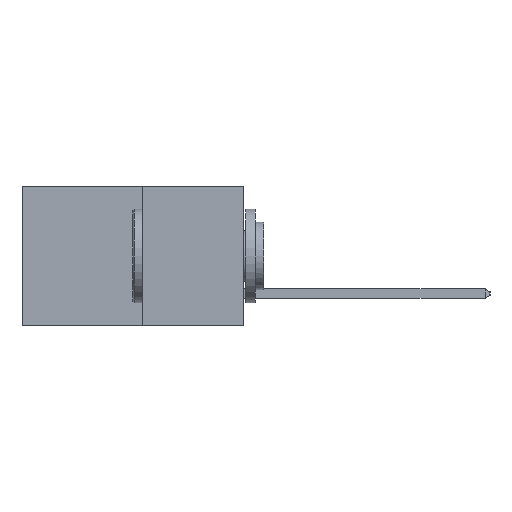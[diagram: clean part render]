
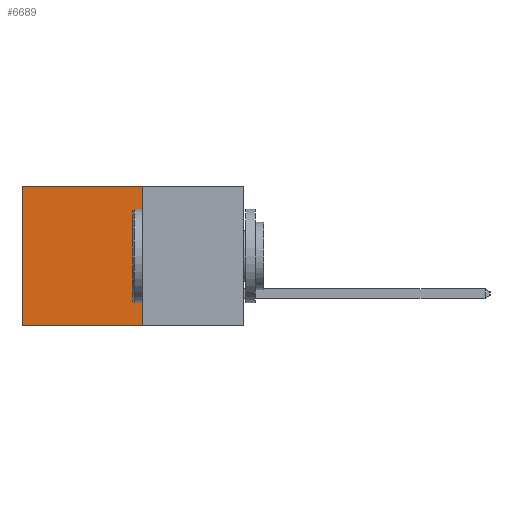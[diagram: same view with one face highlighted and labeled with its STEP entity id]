
A CAD part, left-side view. The second image highlights one B-rep face of the part: STEP entity #6689.
In plain terms, the highlighted planar face has unit normal (-1, 0, 0).
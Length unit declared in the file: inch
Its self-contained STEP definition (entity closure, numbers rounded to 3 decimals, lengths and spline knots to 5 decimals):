
#258 = ORIENTED_EDGE ( 'NONE', *, *, #5710, .T. ) ;
#712 = VERTEX_POINT ( 'NONE', #10095 ) ;
#1313 = VECTOR ( 'NONE', #12692, 39.37008 ) ;
#1452 = CARTESIAN_POINT ( 'NONE',  ( 0.277, 0.27, -0.37 ) ) ;
#1716 = ORIENTED_EDGE ( 'NONE', *, *, #10541, .F. ) ;
#2598 = ORIENTED_EDGE ( 'NONE', *, *, #6685, .F. ) ;
#3275 = VERTEX_POINT ( 'NONE', #8425 ) ;
#3766 = VERTEX_POINT ( 'NONE', #10313 ) ;
#3911 = DIRECTION ( 'NONE',  ( 1., 0., 0. ) ) ;
#4015 = PLANE ( 'NONE',  #11000 ) ;
#4026 = CARTESIAN_POINT ( 'NONE',  ( 0.277, 0.27, -0.37 ) ) ;
#4222 = DIRECTION ( 'NONE',  ( 0., 0., -1. ) ) ;
#4405 = CARTESIAN_POINT ( 'NONE',  ( 0.277, 0.27, -0.37 ) ) ;
#5164 = LINE ( 'NONE', #4405, #10307 ) ;
#5267 = VERTEX_POINT ( 'NONE', #11724 ) ;
#5359 = LINE ( 'NONE', #9083, #7827 ) ;
#5710 = EDGE_CURVE ( 'NONE', #712, #3275, #5359, .T. ) ;
#6685 = EDGE_CURVE ( 'NONE', #5267, #3766, #5164, .T. ) ;
#6689 = ADVANCED_FACE ( 'NONE', ( #12593 ), #4015, .F. ) ;
#6745 = DIRECTION ( 'NONE',  ( 0., 0., -1. ) ) ;
#6902 = LINE ( 'NONE', #12719, #9647 ) ;
#7827 = VECTOR ( 'NONE', #9315, 39.37008 ) ;
#7901 = EDGE_LOOP ( 'NONE', ( #258, #1716, #2598, #11240 ) ) ;
#8425 = CARTESIAN_POINT ( 'NONE',  ( 0.277, 0.59, -0.37 ) ) ;
#9083 = CARTESIAN_POINT ( 'NONE',  ( 0.277, 0.59, -0.37 ) ) ;
#9272 = EDGE_CURVE ( 'NONE', #5267, #712, #6902, .T. ) ;
#9315 = DIRECTION ( 'NONE',  ( 0., 0., -1. ) ) ;
#9610 = LINE ( 'NONE', #1452, #1313 ) ;
#9647 = VECTOR ( 'NONE', #10763, 39.37008 ) ;
#10095 = CARTESIAN_POINT ( 'NONE',  ( 0.277, 0.59, 0. ) ) ;
#10307 = VECTOR ( 'NONE', #4222, 39.37008 ) ;
#10313 = CARTESIAN_POINT ( 'NONE',  ( 0.277, 0.27, -0.37 ) ) ;
#10541 = EDGE_CURVE ( 'NONE', #3766, #3275, #9610, .T. ) ;
#10763 = DIRECTION ( 'NONE',  ( 0., 1., 0. ) ) ;
#11000 = AXIS2_PLACEMENT_3D ( 'NONE', #4026, #3911, #6745 ) ;
#11240 = ORIENTED_EDGE ( 'NONE', *, *, #9272, .T. ) ;
#11724 = CARTESIAN_POINT ( 'NONE',  ( 0.277, 0.27, 0. ) ) ;
#12593 = FACE_OUTER_BOUND ( 'NONE', #7901, .T. ) ;
#12692 = DIRECTION ( 'NONE',  ( 0., 1., 0. ) ) ;
#12719 = CARTESIAN_POINT ( 'NONE',  ( 0.277, 0.27, 0. ) ) ;
